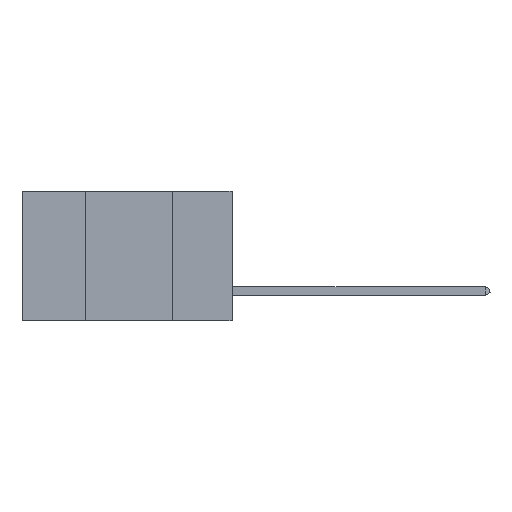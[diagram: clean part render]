
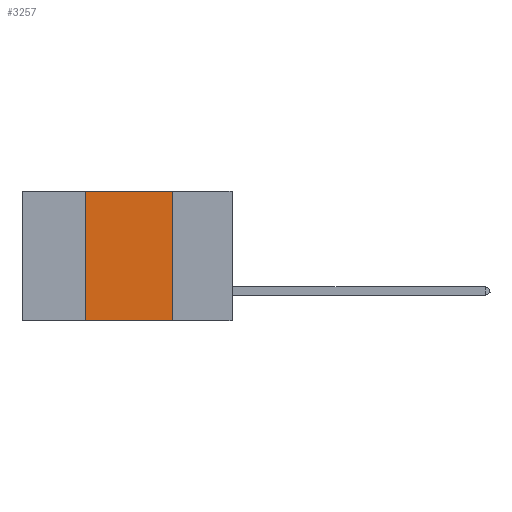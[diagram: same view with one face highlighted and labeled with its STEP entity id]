
A CAD part, left-side view. The second image highlights one B-rep face of the part: STEP entity #3257.
In plain terms, the highlighted planar face has unit normal (-1, 0, 0).
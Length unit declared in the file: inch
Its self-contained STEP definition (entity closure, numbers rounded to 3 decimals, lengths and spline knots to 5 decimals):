
#519 = ORIENTED_EDGE ( 'NONE', *, *, #12607, .F. ) ;
#674 = CARTESIAN_POINT ( 'NONE',  ( 0., 0.17, 0. ) ) ;
#707 = VECTOR ( 'NONE', #17262, 39.37008 ) ;
#849 = EDGE_CURVE ( 'NONE', #5870, #9961, #5629, .T. ) ;
#1971 = LINE ( 'NONE', #5302, #707 ) ;
#2923 = PLANE ( 'NONE',  #14837 ) ;
#3143 = EDGE_CURVE ( 'NONE', #10752, #5870, #5318, .T. ) ;
#3257 = ADVANCED_FACE ( 'NONE', ( #6550 ), #2923, .F. ) ;
#5302 = CARTESIAN_POINT ( 'NONE',  ( 0., 0.6, -0.37 ) ) ;
#5318 = LINE ( 'NONE', #6514, #7186 ) ;
#5629 = LINE ( 'NONE', #674, #15830 ) ;
#5870 = VERTEX_POINT ( 'NONE', #15118 ) ;
#6033 = DIRECTION ( 'NONE',  ( 0., 0., -1. ) ) ;
#6172 = ORIENTED_EDGE ( 'NONE', *, *, #849, .F. ) ;
#6514 = CARTESIAN_POINT ( 'NONE',  ( 0., 0.6, 0. ) ) ;
#6550 = FACE_OUTER_BOUND ( 'NONE', #15292, .T. ) ;
#6627 = DIRECTION ( 'NONE',  ( 0., 0., -1. ) ) ;
#6847 = CARTESIAN_POINT ( 'NONE',  ( 0., 0.6, 0. ) ) ;
#6916 = CARTESIAN_POINT ( 'NONE',  ( 0., 0.42, -0.37 ) ) ;
#7186 = VECTOR ( 'NONE', #15719, 39.37008 ) ;
#7897 = EDGE_CURVE ( 'NONE', #14650, #9961, #1971, .T. ) ;
#8333 = ORIENTED_EDGE ( 'NONE', *, *, #3143, .F. ) ;
#9563 = LINE ( 'NONE', #13995, #14592 ) ;
#9961 = VERTEX_POINT ( 'NONE', #15296 ) ;
#10752 = VERTEX_POINT ( 'NONE', #13231 ) ;
#12055 = ORIENTED_EDGE ( 'NONE', *, *, #7897, .T. ) ;
#12607 = EDGE_CURVE ( 'NONE', #14650, #10752, #9563, .T. ) ;
#12886 = DIRECTION ( 'NONE',  ( 0., 0., 1. ) ) ;
#13231 = CARTESIAN_POINT ( 'NONE',  ( 0., 0.42, 0. ) ) ;
#13995 = CARTESIAN_POINT ( 'NONE',  ( 0., 0.42, 0. ) ) ;
#14592 = VECTOR ( 'NONE', #12886, 39.37008 ) ;
#14650 = VERTEX_POINT ( 'NONE', #6916 ) ;
#14837 = AXIS2_PLACEMENT_3D ( 'NONE', #6847, #16169, #6627 ) ;
#15118 = CARTESIAN_POINT ( 'NONE',  ( 0., 0.17, 0. ) ) ;
#15292 = EDGE_LOOP ( 'NONE', ( #6172, #8333, #519, #12055 ) ) ;
#15296 = CARTESIAN_POINT ( 'NONE',  ( 0., 0.17, -0.37 ) ) ;
#15719 = DIRECTION ( 'NONE',  ( 0., -1., 0. ) ) ;
#15830 = VECTOR ( 'NONE', #6033, 39.37008 ) ;
#16169 = DIRECTION ( 'NONE',  ( 1., 0., 0. ) ) ;
#17262 = DIRECTION ( 'NONE',  ( 0., -1., 0. ) ) ;
